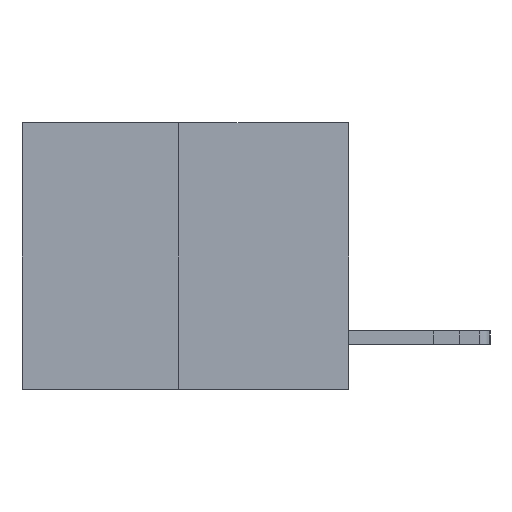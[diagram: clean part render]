
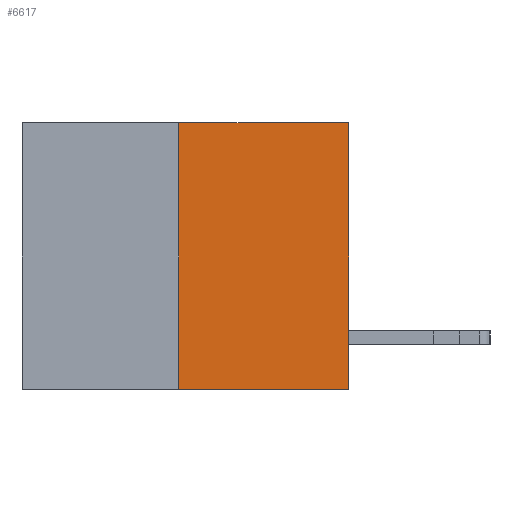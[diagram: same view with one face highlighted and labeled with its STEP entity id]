
A CAD part, left-side view. The second image highlights one B-rep face of the part: STEP entity #6617.
In plain terms, the highlighted planar face has unit normal (-1, 0, 0).
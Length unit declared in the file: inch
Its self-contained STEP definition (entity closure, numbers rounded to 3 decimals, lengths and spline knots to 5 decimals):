
#484 = VECTOR ( 'NONE', #12787, 39.37008 ) ;
#1112 = LINE ( 'NONE', #4245, #7991 ) ;
#1220 = VECTOR ( 'NONE', #9089, 39.37008 ) ;
#1265 = CARTESIAN_POINT ( 'NONE',  ( 0., 0.6, -0.49 ) ) ;
#1438 = CARTESIAN_POINT ( 'NONE',  ( 0., 0.312, 0. ) ) ;
#2353 = DIRECTION ( 'NONE',  ( 0., -1., 0. ) ) ;
#2491 = VERTEX_POINT ( 'NONE', #1438 ) ;
#2615 = CARTESIAN_POINT ( 'NONE',  ( 0., 0.312, -0.49 ) ) ;
#2954 = VERTEX_POINT ( 'NONE', #10623 ) ;
#3061 = VECTOR ( 'NONE', #2353, 39.37008 ) ;
#3232 = LINE ( 'NONE', #11743, #484 ) ;
#3803 = ORIENTED_EDGE ( 'NONE', *, *, #7204, .F. ) ;
#4245 = CARTESIAN_POINT ( 'NONE',  ( 0., 0., 0. ) ) ;
#4955 = LINE ( 'NONE', #1265, #3061 ) ;
#5087 = EDGE_CURVE ( 'NONE', #10585, #2954, #1112, .T. ) ;
#5363 = DIRECTION ( 'NONE',  ( 0., 0., 1. ) ) ;
#5618 = CARTESIAN_POINT ( 'NONE',  ( 0., 0.312, -0.49 ) ) ;
#5991 = AXIS2_PLACEMENT_3D ( 'NONE', #7367, #10633, #8827 ) ;
#6133 = ORIENTED_EDGE ( 'NONE', *, *, #8790, .F. ) ;
#6435 = CARTESIAN_POINT ( 'NONE',  ( 0., 0., -0.49 ) ) ;
#6617 = ADVANCED_FACE ( 'NONE', ( #10750 ), #12893, .F. ) ;
#7204 = EDGE_CURVE ( 'NONE', #8491, #2491, #7583, .T. ) ;
#7367 = CARTESIAN_POINT ( 'NONE',  ( 0., 0.6, 0. ) ) ;
#7583 = LINE ( 'NONE', #2615, #1220 ) ;
#7991 = VECTOR ( 'NONE', #5363, 39.37008 ) ;
#8399 = EDGE_CURVE ( 'NONE', #8491, #10585, #4955, .T. ) ;
#8491 = VERTEX_POINT ( 'NONE', #5618 ) ;
#8790 = EDGE_CURVE ( 'NONE', #2491, #2954, #3232, .T. ) ;
#8827 = DIRECTION ( 'NONE',  ( 0., 0., -1. ) ) ;
#9089 = DIRECTION ( 'NONE',  ( 0., 0., 1. ) ) ;
#10585 = VERTEX_POINT ( 'NONE', #6435 ) ;
#10623 = CARTESIAN_POINT ( 'NONE',  ( 0., 0., 0. ) ) ;
#10633 = DIRECTION ( 'NONE',  ( 1., 0., 0. ) ) ;
#10750 = FACE_OUTER_BOUND ( 'NONE', #11222, .T. ) ;
#11222 = EDGE_LOOP ( 'NONE', ( #3803, #12437, #12777, #6133 ) ) ;
#11743 = CARTESIAN_POINT ( 'NONE',  ( 0., 0.6, 0. ) ) ;
#12437 = ORIENTED_EDGE ( 'NONE', *, *, #8399, .T. ) ;
#12777 = ORIENTED_EDGE ( 'NONE', *, *, #5087, .T. ) ;
#12787 = DIRECTION ( 'NONE',  ( 0., -1., 0. ) ) ;
#12893 = PLANE ( 'NONE',  #5991 ) ;
